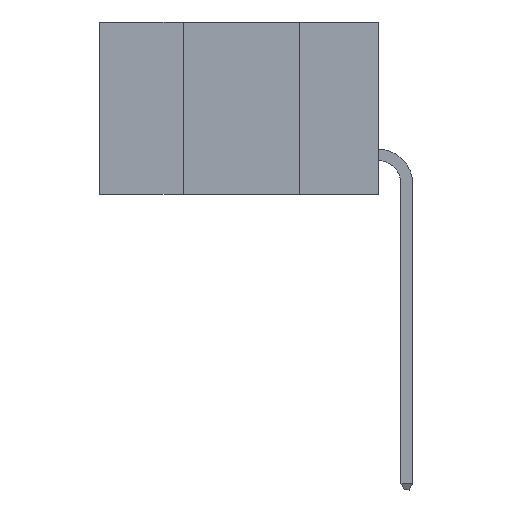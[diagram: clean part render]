
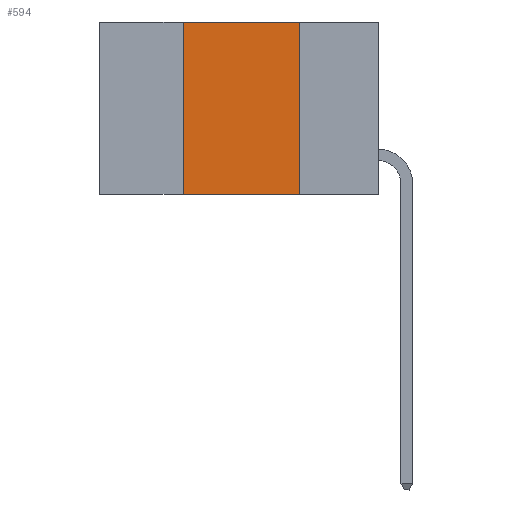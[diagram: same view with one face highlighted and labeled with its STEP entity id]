
A CAD part, left-side view. The second image highlights one B-rep face of the part: STEP entity #594.
In plain terms, the highlighted planar face has unit normal (-1, 0, 0).
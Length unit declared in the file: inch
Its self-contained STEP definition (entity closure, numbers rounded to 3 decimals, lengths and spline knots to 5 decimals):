
#332 = DIRECTION ( 'NONE',  ( 0., 0., 1. ) ) ;
#543 = EDGE_CURVE ( 'NONE', #10791, #12806, #5571, .T. ) ;
#594 = ADVANCED_FACE ( 'NONE', ( #2892 ), #11819, .F. ) ;
#747 = EDGE_CURVE ( 'NONE', #8230, #10791, #1840, .T. ) ;
#1539 = EDGE_CURVE ( 'NONE', #6190, #12806, #12679, .T. ) ;
#1825 = DIRECTION ( 'NONE',  ( 0., 0., -1. ) ) ;
#1840 = LINE ( 'NONE', #12716, #11072 ) ;
#2892 = FACE_OUTER_BOUND ( 'NONE', #7236, .T. ) ;
#3648 = CARTESIAN_POINT ( 'NONE',  ( 0., 0.17, 0. ) ) ;
#4499 = CARTESIAN_POINT ( 'NONE',  ( 0., 0.6, -0.37 ) ) ;
#4912 = ORIENTED_EDGE ( 'NONE', *, *, #8631, .F. ) ;
#5510 = DIRECTION ( 'NONE',  ( 0., -1., 0. ) ) ;
#5571 = LINE ( 'NONE', #3648, #7247 ) ;
#6190 = VERTEX_POINT ( 'NONE', #6960 ) ;
#6960 = CARTESIAN_POINT ( 'NONE',  ( 0., 0.42, -0.37 ) ) ;
#7236 = EDGE_LOOP ( 'NONE', ( #12088, #8698, #4912, #11485 ) ) ;
#7247 = VECTOR ( 'NONE', #11445, 39.37008 ) ;
#8130 = CARTESIAN_POINT ( 'NONE',  ( 0., 0.42, 0. ) ) ;
#8230 = VERTEX_POINT ( 'NONE', #8130 ) ;
#8631 = EDGE_CURVE ( 'NONE', #6190, #8230, #9915, .T. ) ;
#8698 = ORIENTED_EDGE ( 'NONE', *, *, #747, .F. ) ;
#9747 = DIRECTION ( 'NONE',  ( 1., 0., 0. ) ) ;
#9753 = VECTOR ( 'NONE', #332, 39.37008 ) ;
#9794 = CARTESIAN_POINT ( 'NONE',  ( 0., 0.6, 0. ) ) ;
#9915 = LINE ( 'NONE', #12222, #9753 ) ;
#10791 = VERTEX_POINT ( 'NONE', #11119 ) ;
#10909 = AXIS2_PLACEMENT_3D ( 'NONE', #9794, #9747, #1825 ) ;
#11072 = VECTOR ( 'NONE', #11962, 39.37008 ) ;
#11119 = CARTESIAN_POINT ( 'NONE',  ( 0., 0.17, 0. ) ) ;
#11445 = DIRECTION ( 'NONE',  ( 0., 0., -1. ) ) ;
#11485 = ORIENTED_EDGE ( 'NONE', *, *, #1539, .T. ) ;
#11819 = PLANE ( 'NONE',  #10909 ) ;
#11861 = VECTOR ( 'NONE', #5510, 39.37008 ) ;
#11871 = CARTESIAN_POINT ( 'NONE',  ( 0., 0.17, -0.37 ) ) ;
#11962 = DIRECTION ( 'NONE',  ( 0., -1., 0. ) ) ;
#12088 = ORIENTED_EDGE ( 'NONE', *, *, #543, .F. ) ;
#12222 = CARTESIAN_POINT ( 'NONE',  ( 0., 0.42, 0. ) ) ;
#12679 = LINE ( 'NONE', #4499, #11861 ) ;
#12716 = CARTESIAN_POINT ( 'NONE',  ( 0., 0.6, 0. ) ) ;
#12806 = VERTEX_POINT ( 'NONE', #11871 ) ;
